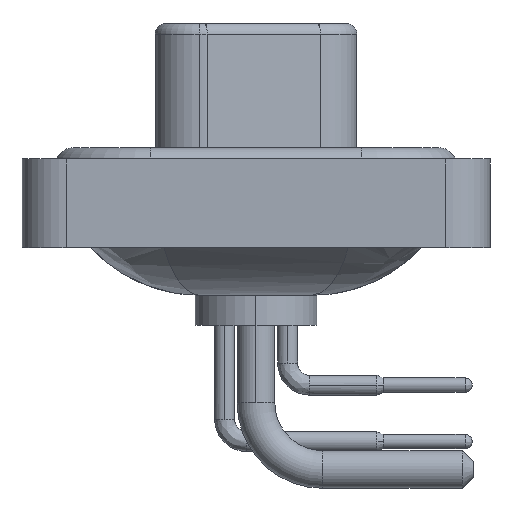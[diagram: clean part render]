
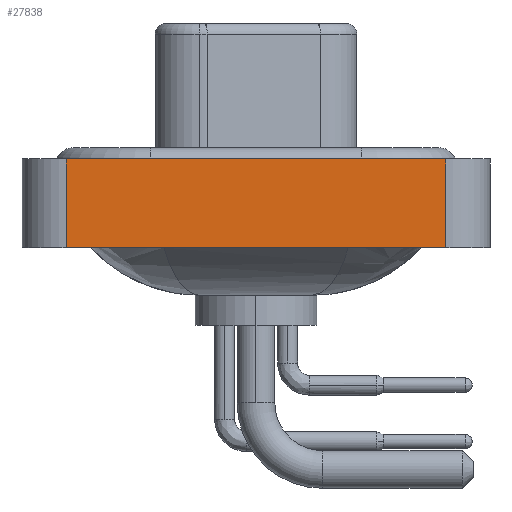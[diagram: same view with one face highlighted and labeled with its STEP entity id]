
A CAD part, left-side view. The second image highlights one B-rep face of the part: STEP entity #27838.
In plain terms, the highlighted planar face has unit normal (-1, 0, 0).
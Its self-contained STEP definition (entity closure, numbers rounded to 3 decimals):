
#20 = EDGE_CURVE ( 'NONE', #21761, #1724, #17300, .T. ) ;
#1724 = VERTEX_POINT ( 'NONE', #23714 ) ;
#2055 = DIRECTION ( 'NONE',  ( 0., -1., 0. ) ) ;
#3850 = VERTEX_POINT ( 'NONE', #10762 ) ;
#4200 = ORIENTED_EDGE ( 'NONE', *, *, #23220, .T. ) ;
#4373 = CARTESIAN_POINT ( 'NONE',  ( -7.35, 8.55, -3.6 ) ) ;
#5077 = VECTOR ( 'NONE', #16268, 1000. ) ;
#5935 = ORIENTED_EDGE ( 'NONE', *, *, #15458, .F. ) ;
#7122 = VECTOR ( 'NONE', #17239, 1000. ) ;
#7292 = CARTESIAN_POINT ( 'NONE',  ( -7.35, -8.55, -3.6 ) ) ;
#7574 = PLANE ( 'NONE',  #16494 ) ;
#10762 = CARTESIAN_POINT ( 'NONE',  ( -7.35, -8.55, -3.6 ) ) ;
#11225 = CARTESIAN_POINT ( 'NONE',  ( -7.35, -8.55, 0.4 ) ) ;
#11645 = EDGE_CURVE ( 'NONE', #21761, #3850, #13216, .T. ) ;
#11973 = LINE ( 'NONE', #23188, #5077 ) ;
#12451 = ORIENTED_EDGE ( 'NONE', *, *, #11645, .T. ) ;
#13216 = LINE ( 'NONE', #21856, #7122 ) ;
#13893 = EDGE_LOOP ( 'NONE', ( #4200, #5935, #26332, #12451 ) ) ;
#15458 = EDGE_CURVE ( 'NONE', #1724, #22196, #17274, .T. ) ;
#16268 = DIRECTION ( 'NONE',  ( 0., 0., 1. ) ) ;
#16494 = AXIS2_PLACEMENT_3D ( 'NONE', #7292, #22660, #20505 ) ;
#17239 = DIRECTION ( 'NONE',  ( 0., -1., 0. ) ) ;
#17274 = LINE ( 'NONE', #11225, #24312 ) ;
#17300 = LINE ( 'NONE', #4373, #27529 ) ;
#17835 = CARTESIAN_POINT ( 'NONE',  ( -7.35, 8.55, -3.6 ) ) ;
#20505 = DIRECTION ( 'NONE',  ( 0., 0., 1. ) ) ;
#21426 = CARTESIAN_POINT ( 'NONE',  ( -7.35, -8.55, 0.4 ) ) ;
#21761 = VERTEX_POINT ( 'NONE', #17835 ) ;
#21856 = CARTESIAN_POINT ( 'NONE',  ( -7.35, -8.55, -3.6 ) ) ;
#21913 = DIRECTION ( 'NONE',  ( 0., 0., 1. ) ) ;
#22196 = VERTEX_POINT ( 'NONE', #21426 ) ;
#22660 = DIRECTION ( 'NONE',  ( -1., 0., 0. ) ) ;
#23188 = CARTESIAN_POINT ( 'NONE',  ( -7.35, -8.55, -3.6 ) ) ;
#23220 = EDGE_CURVE ( 'NONE', #3850, #22196, #11973, .T. ) ;
#23714 = CARTESIAN_POINT ( 'NONE',  ( -7.35, 8.55, 0.4 ) ) ;
#24312 = VECTOR ( 'NONE', #2055, 1000. ) ;
#26332 = ORIENTED_EDGE ( 'NONE', *, *, #20, .F. ) ;
#26955 = FACE_OUTER_BOUND ( 'NONE', #13893, .T. ) ;
#27529 = VECTOR ( 'NONE', #21913, 1000. ) ;
#27838 = ADVANCED_FACE ( 'NONE', ( #26955 ), #7574, .T. ) ;
